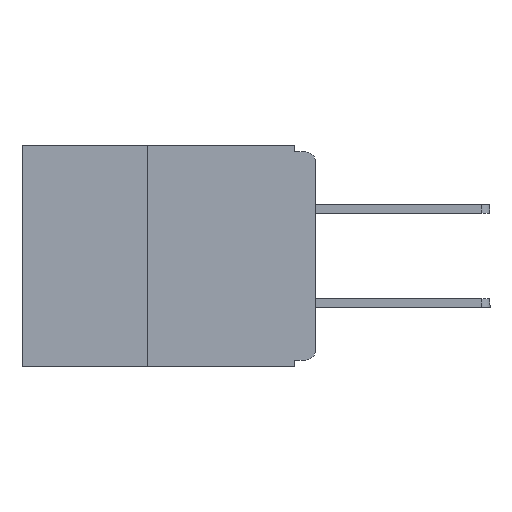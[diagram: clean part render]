
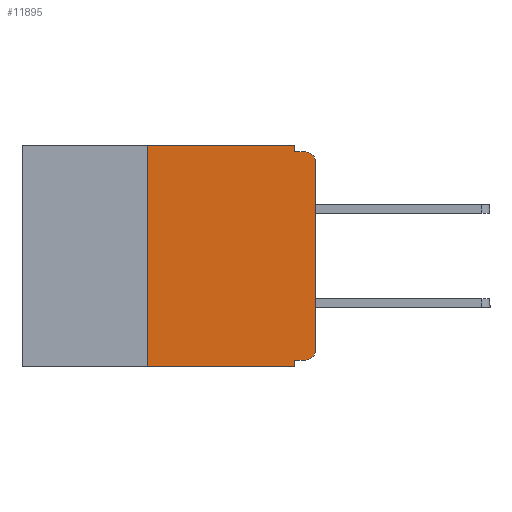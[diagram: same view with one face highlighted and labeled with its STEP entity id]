
A CAD part, left-side view. The second image highlights one B-rep face of the part: STEP entity #11895.
In plain terms, the highlighted planar face has unit normal (-1, 0, 0).
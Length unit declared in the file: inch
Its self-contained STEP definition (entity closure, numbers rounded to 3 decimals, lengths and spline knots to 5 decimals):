
#238 = VECTOR ( 'NONE', #4777, 39.37008 ) ;
#510 = CARTESIAN_POINT ( 'NONE',  ( 0., 0.437, 0. ) ) ;
#529 = VECTOR ( 'NONE', #1327, 39.37008 ) ;
#542 = LINE ( 'NONE', #4904, #238 ) ;
#633 = ORIENTED_EDGE ( 'NONE', *, *, #11185, .T. ) ;
#739 = DIRECTION ( 'NONE',  ( 0., 0., 1. ) ) ;
#793 = CARTESIAN_POINT ( 'NONE',  ( 0., 0.25, -0.33 ) ) ;
#1050 = VERTEX_POINT ( 'NONE', #4310 ) ;
#1247 = VECTOR ( 'NONE', #739, 39.37008 ) ;
#1327 = DIRECTION ( 'NONE',  ( 0., -1., 0. ) ) ;
#1500 = DIRECTION ( 'NONE',  ( 0., 0., -1. ) ) ;
#1509 = LINE ( 'NONE', #11061, #6189 ) ;
#1672 = ORIENTED_EDGE ( 'NONE', *, *, #10984, .F. ) ;
#1698 = EDGE_CURVE ( 'NONE', #1050, #2330, #1914, .T. ) ;
#1906 = CARTESIAN_POINT ( 'NONE',  ( 0., 0.437, 0. ) ) ;
#1914 = LINE ( 'NONE', #5801, #6831 ) ;
#1998 = DIRECTION ( 'NONE',  ( 0., 0., 1. ) ) ;
#2242 = ORIENTED_EDGE ( 'NONE', *, *, #8479, .T. ) ;
#2330 = VERTEX_POINT ( 'NONE', #9508 ) ;
#2539 = VERTEX_POINT ( 'NONE', #3473 ) ;
#2927 = CARTESIAN_POINT ( 'NONE',  ( 0., 0.015, -0.01 ) ) ;
#2950 = LINE ( 'NONE', #6232, #7532 ) ;
#3296 = VERTEX_POINT ( 'NONE', #11229 ) ;
#3348 = DIRECTION ( 'NONE',  ( -1., 0., 0. ) ) ;
#3389 = CARTESIAN_POINT ( 'NONE',  ( 0., 0.031, -0.33 ) ) ;
#3458 = ORIENTED_EDGE ( 'NONE', *, *, #7381, .F. ) ;
#3465 = FACE_OUTER_BOUND ( 'NONE', #7501, .T. ) ;
#3473 = CARTESIAN_POINT ( 'NONE',  ( 0., 0.015, -0.32 ) ) ;
#3488 = CARTESIAN_POINT ( 'NONE',  ( 0., 0.031, 0. ) ) ;
#3615 = AXIS2_PLACEMENT_3D ( 'NONE', #9768, #4269, #10717 ) ;
#3774 = LINE ( 'NONE', #793, #1247 ) ;
#3954 = EDGE_CURVE ( 'NONE', #3296, #7840, #6595, .T. ) ;
#4190 = EDGE_CURVE ( 'NONE', #10139, #6374, #1509, .T. ) ;
#4258 = DIRECTION ( 'NONE',  ( 0., -1., 0. ) ) ;
#4269 = DIRECTION ( 'NONE',  ( -1., 0., 0. ) ) ;
#4294 = CARTESIAN_POINT ( 'NONE',  ( 0., 0.437, -0.33 ) ) ;
#4310 = CARTESIAN_POINT ( 'NONE',  ( 0., 0., -0.305 ) ) ;
#4392 = ORIENTED_EDGE ( 'NONE', *, *, #7156, .F. ) ;
#4398 = LINE ( 'NONE', #4294, #6549 ) ;
#4551 = ORIENTED_EDGE ( 'NONE', *, *, #8397, .F. ) ;
#4777 = DIRECTION ( 'NONE',  ( 0., -1., 0. ) ) ;
#4892 = VERTEX_POINT ( 'NONE', #2927 ) ;
#4904 = CARTESIAN_POINT ( 'NONE',  ( 0., 0., -0.01 ) ) ;
#5148 = ORIENTED_EDGE ( 'NONE', *, *, #11855, .T. ) ;
#5553 = LINE ( 'NONE', #1906, #529 ) ;
#5784 = CIRCLE ( 'NONE', #9212, 0.015 ) ;
#5801 = CARTESIAN_POINT ( 'NONE',  ( 0., 0., 0. ) ) ;
#6042 = DIRECTION ( 'NONE',  ( 0., 1., 0. ) ) ;
#6156 = PLANE ( 'NONE',  #6656 ) ;
#6189 = VECTOR ( 'NONE', #7146, 39.37008 ) ;
#6232 = CARTESIAN_POINT ( 'NONE',  ( 0., 0., -0.32 ) ) ;
#6360 = ORIENTED_EDGE ( 'NONE', *, *, #3954, .F. ) ;
#6374 = VERTEX_POINT ( 'NONE', #3389 ) ;
#6549 = VECTOR ( 'NONE', #4258, 39.37008 ) ;
#6595 = LINE ( 'NONE', #3488, #8764 ) ;
#6623 = ORIENTED_EDGE ( 'NONE', *, *, #1698, .T. ) ;
#6656 = AXIS2_PLACEMENT_3D ( 'NONE', #510, #7062, #1500 ) ;
#6831 = VECTOR ( 'NONE', #1998, 39.37008 ) ;
#7062 = DIRECTION ( 'NONE',  ( 1., 0., 0. ) ) ;
#7146 = DIRECTION ( 'NONE',  ( 0., 0., -1. ) ) ;
#7156 = EDGE_CURVE ( 'NONE', #2539, #10139, #2950, .T. ) ;
#7381 = EDGE_CURVE ( 'NONE', #7806, #3296, #5553, .T. ) ;
#7501 = EDGE_LOOP ( 'NONE', ( #6623, #5148, #4551, #6360, #3458, #1672, #2242, #8363, #4392, #633 ) ) ;
#7532 = VECTOR ( 'NONE', #6042, 39.37008 ) ;
#7806 = VERTEX_POINT ( 'NONE', #9646 ) ;
#7840 = VERTEX_POINT ( 'NONE', #9130 ) ;
#8220 = CARTESIAN_POINT ( 'NONE',  ( 0., 0.031, -0.32 ) ) ;
#8330 = CIRCLE ( 'NONE', #3615, 0.015 ) ;
#8363 = ORIENTED_EDGE ( 'NONE', *, *, #4190, .F. ) ;
#8397 = EDGE_CURVE ( 'NONE', #7840, #4892, #542, .T. ) ;
#8479 = EDGE_CURVE ( 'NONE', #9829, #6374, #4398, .T. ) ;
#8764 = VECTOR ( 'NONE', #11716, 39.37008 ) ;
#8836 = CARTESIAN_POINT ( 'NONE',  ( 0., 0.015, -0.305 ) ) ;
#9130 = CARTESIAN_POINT ( 'NONE',  ( 0., 0.031, -0.01 ) ) ;
#9212 = AXIS2_PLACEMENT_3D ( 'NONE', #8836, #3348, #9780 ) ;
#9508 = CARTESIAN_POINT ( 'NONE',  ( 0., 0., -0.025 ) ) ;
#9646 = CARTESIAN_POINT ( 'NONE',  ( 0., 0.25, 0. ) ) ;
#9768 = CARTESIAN_POINT ( 'NONE',  ( 0., 0.015, -0.025 ) ) ;
#9780 = DIRECTION ( 'NONE',  ( 0., 0., -1. ) ) ;
#9829 = VERTEX_POINT ( 'NONE', #10751 ) ;
#10139 = VERTEX_POINT ( 'NONE', #8220 ) ;
#10717 = DIRECTION ( 'NONE',  ( 0., 0., -1. ) ) ;
#10751 = CARTESIAN_POINT ( 'NONE',  ( 0., 0.25, -0.33 ) ) ;
#10984 = EDGE_CURVE ( 'NONE', #9829, #7806, #3774, .T. ) ;
#11061 = CARTESIAN_POINT ( 'NONE',  ( 0., 0.031, -0.33 ) ) ;
#11185 = EDGE_CURVE ( 'NONE', #2539, #1050, #5784, .T. ) ;
#11229 = CARTESIAN_POINT ( 'NONE',  ( 0., 0.031, 0. ) ) ;
#11716 = DIRECTION ( 'NONE',  ( 0., 0., -1. ) ) ;
#11855 = EDGE_CURVE ( 'NONE', #2330, #4892, #8330, .T. ) ;
#11895 = ADVANCED_FACE ( 'NONE', ( #3465 ), #6156, .F. ) ;
